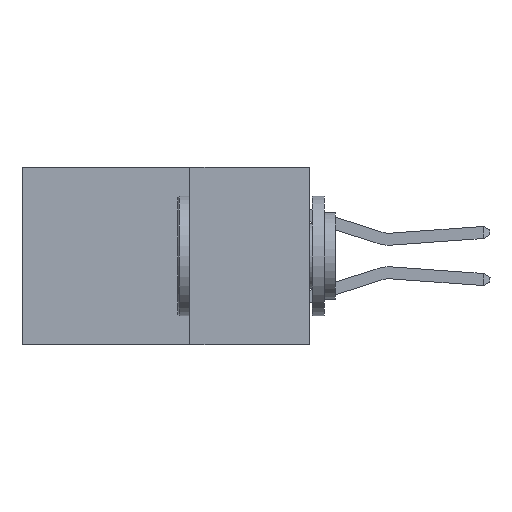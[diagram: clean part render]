
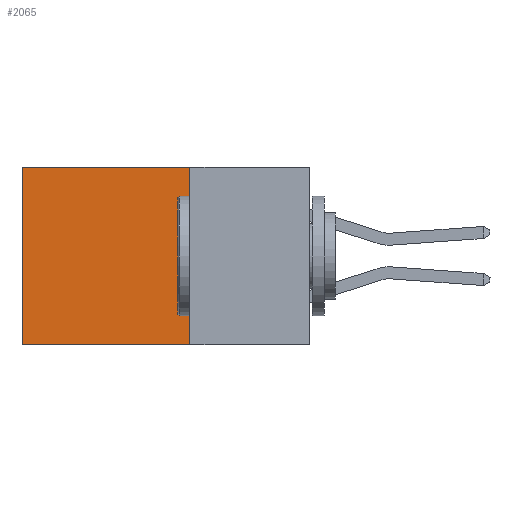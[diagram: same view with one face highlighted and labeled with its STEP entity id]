
A CAD part, left-side view. The second image highlights one B-rep face of the part: STEP entity #2065.
In plain terms, the highlighted planar face has unit normal (-1, 0, 0).
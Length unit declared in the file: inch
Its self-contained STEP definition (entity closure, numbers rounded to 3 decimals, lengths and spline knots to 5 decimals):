
#350 = CARTESIAN_POINT ( 'NONE',  ( 0.2615, 0.6, 0. ) ) ;
#871 = EDGE_CURVE ( 'NONE', #3627, #7821, #1450, .T. ) ;
#1055 = VECTOR ( 'NONE', #6902, 39.37008 ) ;
#1363 = ORIENTED_EDGE ( 'NONE', *, *, #2229, .F. ) ;
#1450 = LINE ( 'NONE', #9386, #1055 ) ;
#1750 = CARTESIAN_POINT ( 'NONE',  ( 0.2615, 0.25, 0. ) ) ;
#1766 = ORIENTED_EDGE ( 'NONE', *, *, #5998, .T. ) ;
#2065 = ADVANCED_FACE ( 'NONE', ( #6365 ), #3767, .F. ) ;
#2229 = EDGE_CURVE ( 'NONE', #3069, #3627, #4709, .T. ) ;
#2488 = DIRECTION ( 'NONE',  ( 0., 1., 0. ) ) ;
#3012 = EDGE_CURVE ( 'NONE', #8455, #7821, #9239, .T. ) ;
#3069 = VERTEX_POINT ( 'NONE', #3244 ) ;
#3083 = DIRECTION ( 'NONE',  ( 1., 0., 0. ) ) ;
#3244 = CARTESIAN_POINT ( 'NONE',  ( 0.2615, 0.25, 0. ) ) ;
#3627 = VERTEX_POINT ( 'NONE', #4330 ) ;
#3767 = PLANE ( 'NONE',  #7962 ) ;
#3803 = CARTESIAN_POINT ( 'NONE',  ( 0.2615, 0.25, -0.37 ) ) ;
#3908 = CARTESIAN_POINT ( 'NONE',  ( 0.2615, 0.6, -0.37 ) ) ;
#3999 = CARTESIAN_POINT ( 'NONE',  ( 0.2615, 0.6, -0.37 ) ) ;
#4017 = ORIENTED_EDGE ( 'NONE', *, *, #3012, .T. ) ;
#4330 = CARTESIAN_POINT ( 'NONE',  ( 0.2615, 0.25, -0.37 ) ) ;
#4709 = LINE ( 'NONE', #4932, #10558 ) ;
#4932 = CARTESIAN_POINT ( 'NONE',  ( 0.2615, 0.25, -0.37 ) ) ;
#4978 = LINE ( 'NONE', #1750, #10432 ) ;
#5421 = EDGE_LOOP ( 'NONE', ( #4017, #7765, #1363, #1766 ) ) ;
#5998 = EDGE_CURVE ( 'NONE', #3069, #8455, #4978, .T. ) ;
#6365 = FACE_OUTER_BOUND ( 'NONE', #5421, .T. ) ;
#6431 = DIRECTION ( 'NONE',  ( 0., 0., -1. ) ) ;
#6902 = DIRECTION ( 'NONE',  ( 0., 1., 0. ) ) ;
#6998 = VECTOR ( 'NONE', #7288, 39.37008 ) ;
#7288 = DIRECTION ( 'NONE',  ( 0., 0., -1. ) ) ;
#7335 = DIRECTION ( 'NONE',  ( 0., 0., -1. ) ) ;
#7765 = ORIENTED_EDGE ( 'NONE', *, *, #871, .F. ) ;
#7821 = VERTEX_POINT ( 'NONE', #3908 ) ;
#7962 = AXIS2_PLACEMENT_3D ( 'NONE', #3803, #3083, #6431 ) ;
#8455 = VERTEX_POINT ( 'NONE', #350 ) ;
#9239 = LINE ( 'NONE', #3999, #6998 ) ;
#9386 = CARTESIAN_POINT ( 'NONE',  ( 0.2615, 0.25, -0.37 ) ) ;
#10432 = VECTOR ( 'NONE', #2488, 39.37008 ) ;
#10558 = VECTOR ( 'NONE', #7335, 39.37008 ) ;
